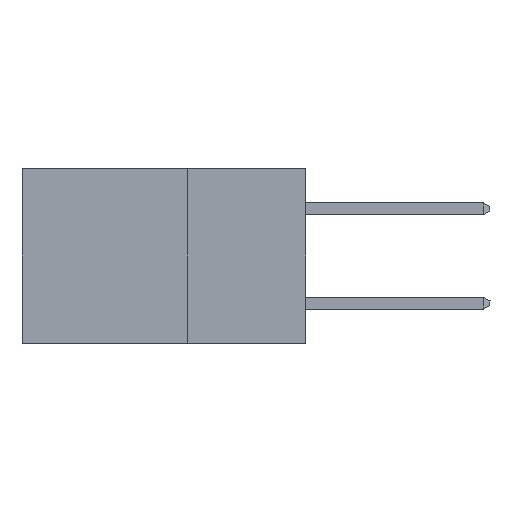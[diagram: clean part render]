
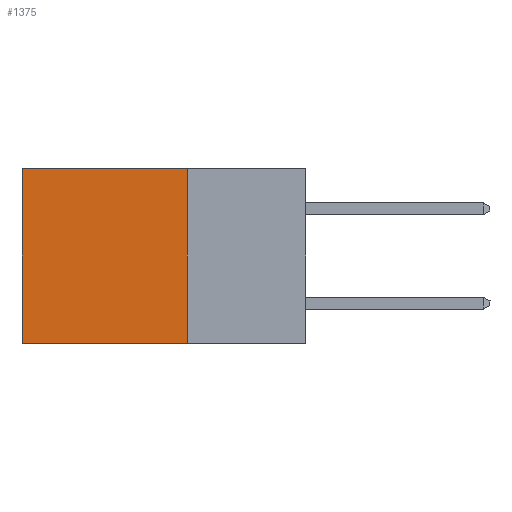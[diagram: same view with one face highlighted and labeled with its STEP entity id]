
A CAD part, left-side view. The second image highlights one B-rep face of the part: STEP entity #1375.
In plain terms, the highlighted planar face has unit normal (-1, 0, 0).
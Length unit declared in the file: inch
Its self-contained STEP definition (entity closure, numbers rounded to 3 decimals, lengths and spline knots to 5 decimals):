
#1217 = EDGE_CURVE ( 'NONE', #3741, #20316, #22806, .T. ) ;
#1339 = EDGE_CURVE ( 'NONE', #9120, #3741, #27495, .T. ) ;
#1375 = ADVANCED_FACE ( 'NONE', ( #1724 ), #8535, .F. ) ;
#1637 = ORIENTED_EDGE ( 'NONE', *, *, #1339, .T. ) ;
#1724 = FACE_OUTER_BOUND ( 'NONE', #14669, .T. ) ;
#2948 = VECTOR ( 'NONE', #25955, 39.37008 ) ;
#3741 = VERTEX_POINT ( 'NONE', #18467 ) ;
#4635 = VECTOR ( 'NONE', #9026, 39.37008 ) ;
#4668 = CARTESIAN_POINT ( 'NONE',  ( 0.298, 0.25, -0.37 ) ) ;
#6924 = ORIENTED_EDGE ( 'NONE', *, *, #11802, .F. ) ;
#7110 = DIRECTION ( 'NONE',  ( 1., 0., 0. ) ) ;
#8300 = ORIENTED_EDGE ( 'NONE', *, *, #12217, .F. ) ;
#8378 = CARTESIAN_POINT ( 'NONE',  ( 0.298, 0.25, 0. ) ) ;
#8535 = PLANE ( 'NONE',  #26920 ) ;
#9026 = DIRECTION ( 'NONE',  ( 0., 1., 0. ) ) ;
#9120 = VERTEX_POINT ( 'NONE', #14867 ) ;
#10565 = VECTOR ( 'NONE', #20497, 39.37008 ) ;
#10838 = DIRECTION ( 'NONE',  ( 0., 0., -1. ) ) ;
#11802 = EDGE_CURVE ( 'NONE', #9120, #18705, #22999, .T. ) ;
#12217 = EDGE_CURVE ( 'NONE', #18705, #20316, #12774, .T. ) ;
#12774 = LINE ( 'NONE', #4668, #4635 ) ;
#14669 = EDGE_LOOP ( 'NONE', ( #17207, #8300, #6924, #1637 ) ) ;
#14867 = CARTESIAN_POINT ( 'NONE',  ( 0.298, 0.25, 0. ) ) ;
#15083 = CARTESIAN_POINT ( 'NONE',  ( 0.298, 0.25, 0. ) ) ;
#17207 = ORIENTED_EDGE ( 'NONE', *, *, #1217, .T. ) ;
#18467 = CARTESIAN_POINT ( 'NONE',  ( 0.298, 0.6, 0. ) ) ;
#18705 = VERTEX_POINT ( 'NONE', #19433 ) ;
#19001 = CARTESIAN_POINT ( 'NONE',  ( 0.298, 0.6, -0.37 ) ) ;
#19433 = CARTESIAN_POINT ( 'NONE',  ( 0.298, 0.25, -0.37 ) ) ;
#20013 = CARTESIAN_POINT ( 'NONE',  ( 0.298, 0.6, 0. ) ) ;
#20316 = VERTEX_POINT ( 'NONE', #19001 ) ;
#20497 = DIRECTION ( 'NONE',  ( 0., 0., -1. ) ) ;
#22806 = LINE ( 'NONE', #20013, #10565 ) ;
#22999 = LINE ( 'NONE', #26049, #2948 ) ;
#23588 = DIRECTION ( 'NONE',  ( 0., 1., 0. ) ) ;
#23815 = VECTOR ( 'NONE', #23588, 39.37008 ) ;
#25955 = DIRECTION ( 'NONE',  ( 0., 0., -1. ) ) ;
#26049 = CARTESIAN_POINT ( 'NONE',  ( 0.298, 0.25, 0. ) ) ;
#26920 = AXIS2_PLACEMENT_3D ( 'NONE', #15083, #7110, #10838 ) ;
#27495 = LINE ( 'NONE', #8378, #23815 ) ;
